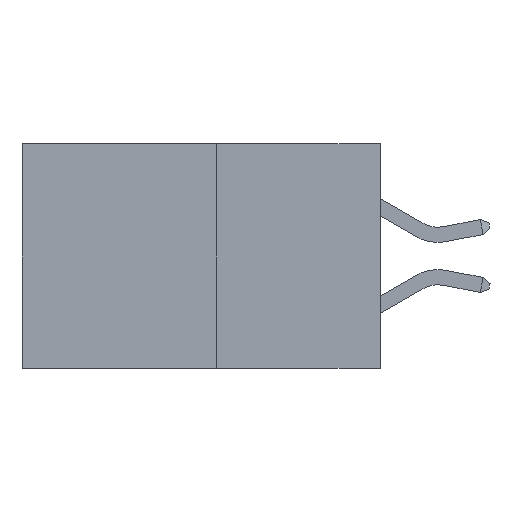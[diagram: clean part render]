
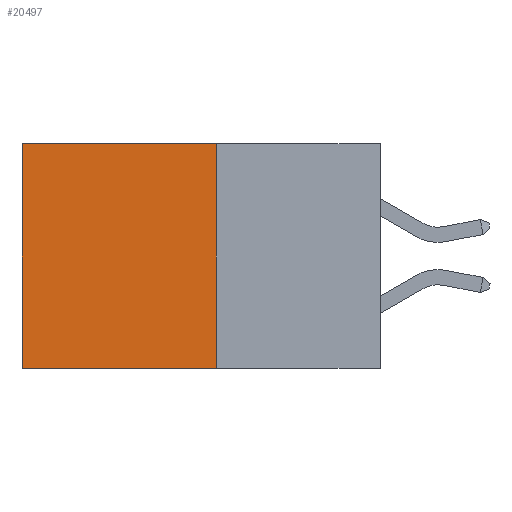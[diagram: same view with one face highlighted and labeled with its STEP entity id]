
A CAD part, left-side view. The second image highlights one B-rep face of the part: STEP entity #20497.
In plain terms, the highlighted planar face has unit normal (-1, 0, 0).
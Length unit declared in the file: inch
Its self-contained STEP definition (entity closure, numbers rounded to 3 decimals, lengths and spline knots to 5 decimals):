
#42 = DIRECTION ( 'NONE',  ( 1., 0., 0. ) ) ;
#1776 = VECTOR ( 'NONE', #7463, 39.37008 ) ;
#2766 = EDGE_CURVE ( 'NONE', #3741, #6850, #5592, .T. ) ;
#3502 = FACE_OUTER_BOUND ( 'NONE', #16328, .T. ) ;
#3741 = VERTEX_POINT ( 'NONE', #11998 ) ;
#5592 = LINE ( 'NONE', #21057, #19652 ) ;
#6285 = EDGE_CURVE ( 'NONE', #22601, #13995, #11337, .T. ) ;
#6850 = VERTEX_POINT ( 'NONE', #8245 ) ;
#7463 = DIRECTION ( 'NONE',  ( 0., 0., -1. ) ) ;
#8245 = CARTESIAN_POINT ( 'NONE',  ( 0.277, 0.27, -0.37 ) ) ;
#8591 = ORIENTED_EDGE ( 'NONE', *, *, #13162, .T. ) ;
#9736 = DIRECTION ( 'NONE',  ( 0., 0., -1. ) ) ;
#10589 = ORIENTED_EDGE ( 'NONE', *, *, #17628, .F. ) ;
#11113 = DIRECTION ( 'NONE',  ( 0., 1., 0. ) ) ;
#11337 = LINE ( 'NONE', #18917, #1776 ) ;
#11476 = CARTESIAN_POINT ( 'NONE',  ( 0.277, 0.27, -0.37 ) ) ;
#11747 = AXIS2_PLACEMENT_3D ( 'NONE', #11476, #42, #13410 ) ;
#11998 = CARTESIAN_POINT ( 'NONE',  ( 0.277, 0.27, 0. ) ) ;
#12459 = CARTESIAN_POINT ( 'NONE',  ( 0.277, 0.59, -0.37 ) ) ;
#12603 = LINE ( 'NONE', #20678, #17640 ) ;
#13162 = EDGE_CURVE ( 'NONE', #3741, #22601, #14421, .T. ) ;
#13410 = DIRECTION ( 'NONE',  ( 0., 0., -1. ) ) ;
#13843 = VECTOR ( 'NONE', #15989, 39.37008 ) ;
#13995 = VERTEX_POINT ( 'NONE', #12459 ) ;
#14421 = LINE ( 'NONE', #19837, #13843 ) ;
#15360 = ORIENTED_EDGE ( 'NONE', *, *, #2766, .F. ) ;
#15989 = DIRECTION ( 'NONE',  ( 0., 1., 0. ) ) ;
#16146 = CARTESIAN_POINT ( 'NONE',  ( 0.277, 0.59, 0. ) ) ;
#16328 = EDGE_LOOP ( 'NONE', ( #20181, #10589, #15360, #8591 ) ) ;
#17628 = EDGE_CURVE ( 'NONE', #6850, #13995, #12603, .T. ) ;
#17640 = VECTOR ( 'NONE', #11113, 39.37008 ) ;
#18917 = CARTESIAN_POINT ( 'NONE',  ( 0.277, 0.59, -0.37 ) ) ;
#19073 = PLANE ( 'NONE',  #11747 ) ;
#19652 = VECTOR ( 'NONE', #9736, 39.37008 ) ;
#19837 = CARTESIAN_POINT ( 'NONE',  ( 0.277, 0.27, 0. ) ) ;
#20181 = ORIENTED_EDGE ( 'NONE', *, *, #6285, .T. ) ;
#20497 = ADVANCED_FACE ( 'NONE', ( #3502 ), #19073, .F. ) ;
#20678 = CARTESIAN_POINT ( 'NONE',  ( 0.277, 0.27, -0.37 ) ) ;
#21057 = CARTESIAN_POINT ( 'NONE',  ( 0.277, 0.27, -0.37 ) ) ;
#22601 = VERTEX_POINT ( 'NONE', #16146 ) ;
